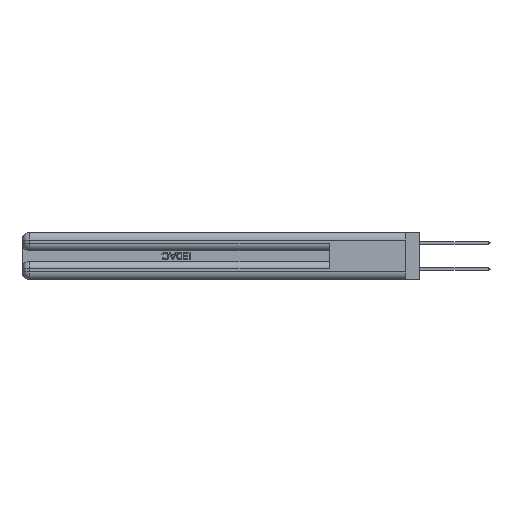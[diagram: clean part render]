
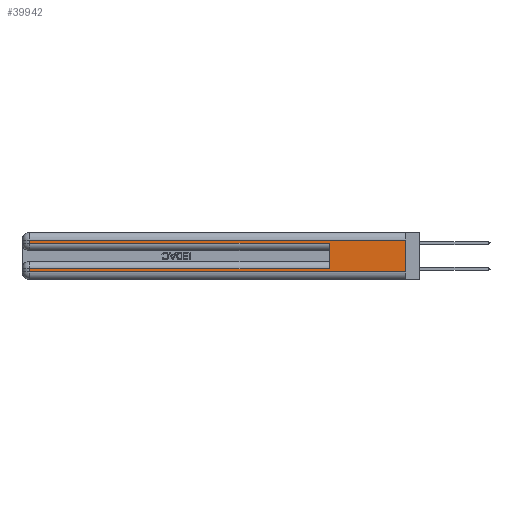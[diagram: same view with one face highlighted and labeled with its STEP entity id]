
A CAD part, left-side view. The second image highlights one B-rep face of the part: STEP entity #39942.
In plain terms, the highlighted planar face has unit normal (-1, 0, 0).
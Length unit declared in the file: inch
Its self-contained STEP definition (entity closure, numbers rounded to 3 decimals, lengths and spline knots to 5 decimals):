
#309 = VECTOR ( 'NONE', #16348, 39.37008 ) ;
#573 = EDGE_CURVE ( 'NONE', #10028, #19249, #5109, .T. ) ;
#2424 = AXIS2_PLACEMENT_3D ( 'NONE', #35760, #16033, #43628 ) ;
#2884 = CARTESIAN_POINT ( 'NONE',  ( 0., 2.94, 0.285 ) ) ;
#2996 = CARTESIAN_POINT ( 'NONE',  ( 0., 2.94, 0.085 ) ) ;
#3483 = EDGE_CURVE ( 'NONE', #23846, #29079, #31442, .T. ) ;
#3544 = DIRECTION ( 'NONE',  ( 0., -1., 0. ) ) ;
#5014 = VECTOR ( 'NONE', #13436, 39.37008 ) ;
#5109 = LINE ( 'NONE', #34774, #35673 ) ;
#7619 = CARTESIAN_POINT ( 'NONE',  ( 0., 2.94, 0.06 ) ) ;
#7771 = VERTEX_POINT ( 'NONE', #2884 ) ;
#9184 = EDGE_CURVE ( 'NONE', #45871, #23846, #19542, .T. ) ;
#9201 = EDGE_CURVE ( 'NONE', #10028, #45871, #48487, .T. ) ;
#10028 = VERTEX_POINT ( 'NONE', #40330 ) ;
#10105 = ORIENTED_EDGE ( 'NONE', *, *, #573, .F. ) ;
#10229 = VECTOR ( 'NONE', #46284, 39.37008 ) ;
#10740 = CARTESIAN_POINT ( 'NONE',  ( 0., 0., 0.06 ) ) ;
#11321 = CARTESIAN_POINT ( 'NONE',  ( 0., 0., 0.31 ) ) ;
#12146 = ORIENTED_EDGE ( 'NONE', *, *, #26129, .T. ) ;
#12360 = LINE ( 'NONE', #36075, #309 ) ;
#13436 = DIRECTION ( 'NONE',  ( 0., 0., -1. ) ) ;
#14805 = ORIENTED_EDGE ( 'NONE', *, *, #25897, .F. ) ;
#15596 = EDGE_LOOP ( 'NONE', ( #14805, #48794, #12146, #17789, #10105, #42801, #37558, #46373 ) ) ;
#16033 = DIRECTION ( 'NONE',  ( 1., 0., 0. ) ) ;
#16348 = DIRECTION ( 'NONE',  ( 0., 1., 0. ) ) ;
#17789 = ORIENTED_EDGE ( 'NONE', *, *, #39212, .T. ) ;
#19009 = DIRECTION ( 'NONE',  ( 0., 0., 1. ) ) ;
#19249 = VERTEX_POINT ( 'NONE', #36043 ) ;
#19542 = LINE ( 'NONE', #22692, #10229 ) ;
#20883 = VECTOR ( 'NONE', #28965, 39.37008 ) ;
#22692 = CARTESIAN_POINT ( 'NONE',  ( 0., 2.94, 0.37 ) ) ;
#23478 = VECTOR ( 'NONE', #30697, 39.37008 ) ;
#23846 = VERTEX_POINT ( 'NONE', #7619 ) ;
#24118 = LINE ( 'NONE', #35467, #33450 ) ;
#24951 = CARTESIAN_POINT ( 'NONE',  ( 0., 0., 0.06 ) ) ;
#25897 = EDGE_CURVE ( 'NONE', #51287, #29079, #45928, .T. ) ;
#26129 = EDGE_CURVE ( 'NONE', #42318, #7771, #44486, .T. ) ;
#26365 = EDGE_CURVE ( 'NONE', #51287, #42318, #12360, .T. ) ;
#26691 = CARTESIAN_POINT ( 'NONE',  ( 0., 2.94, 0.37 ) ) ;
#27606 = VECTOR ( 'NONE', #30853, 39.37008 ) ;
#28965 = DIRECTION ( 'NONE',  ( 0., -1., 0. ) ) ;
#29079 = VERTEX_POINT ( 'NONE', #10740 ) ;
#29130 = CARTESIAN_POINT ( 'NONE',  ( 0., 2.94, 0.31 ) ) ;
#30697 = DIRECTION ( 'NONE',  ( 0., 0., -1. ) ) ;
#30853 = DIRECTION ( 'NONE',  ( 0., 1., 0. ) ) ;
#31442 = LINE ( 'NONE', #24951, #20883 ) ;
#31756 = PLANE ( 'NONE',  #2424 ) ;
#32753 = FACE_OUTER_BOUND ( 'NONE', #15596, .T. ) ;
#33450 = VECTOR ( 'NONE', #3544, 39.37008 ) ;
#34774 = CARTESIAN_POINT ( 'NONE',  ( 0., 0.6, 0.145 ) ) ;
#35467 = CARTESIAN_POINT ( 'NONE',  ( 0., 0., 0.285 ) ) ;
#35673 = VECTOR ( 'NONE', #19009, 39.37008 ) ;
#35760 = CARTESIAN_POINT ( 'NONE',  ( 0., 0., 0.37 ) ) ;
#36043 = CARTESIAN_POINT ( 'NONE',  ( 0., 0.6, 0.285 ) ) ;
#36075 = CARTESIAN_POINT ( 'NONE',  ( 0., 0., 0.31 ) ) ;
#37558 = ORIENTED_EDGE ( 'NONE', *, *, #9184, .T. ) ;
#38655 = CARTESIAN_POINT ( 'NONE',  ( 0., 0., 0.085 ) ) ;
#39212 = EDGE_CURVE ( 'NONE', #7771, #19249, #24118, .T. ) ;
#39942 = ADVANCED_FACE ( 'NONE', ( #32753 ), #31756, .F. ) ;
#40330 = CARTESIAN_POINT ( 'NONE',  ( 0., 0.6, 0.085 ) ) ;
#41105 = CARTESIAN_POINT ( 'NONE',  ( 0., 0., 0.37 ) ) ;
#42318 = VERTEX_POINT ( 'NONE', #29130 ) ;
#42801 = ORIENTED_EDGE ( 'NONE', *, *, #9201, .T. ) ;
#43628 = DIRECTION ( 'NONE',  ( 0., 0., -1. ) ) ;
#44486 = LINE ( 'NONE', #26691, #23478 ) ;
#45871 = VERTEX_POINT ( 'NONE', #2996 ) ;
#45928 = LINE ( 'NONE', #41105, #5014 ) ;
#46284 = DIRECTION ( 'NONE',  ( 0., 0., -1. ) ) ;
#46373 = ORIENTED_EDGE ( 'NONE', *, *, #3483, .T. ) ;
#48487 = LINE ( 'NONE', #38655, #27606 ) ;
#48794 = ORIENTED_EDGE ( 'NONE', *, *, #26365, .T. ) ;
#51287 = VERTEX_POINT ( 'NONE', #11321 ) ;
